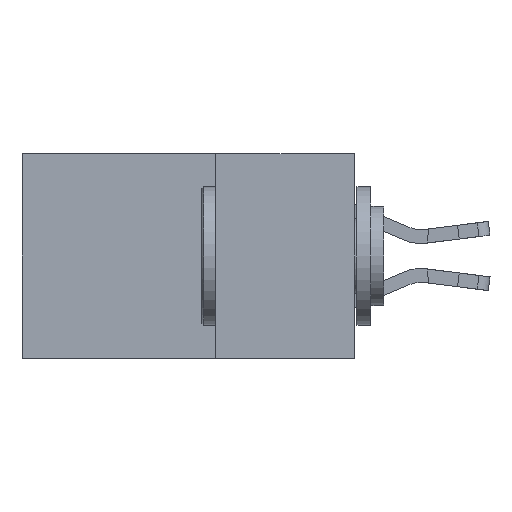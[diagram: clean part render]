
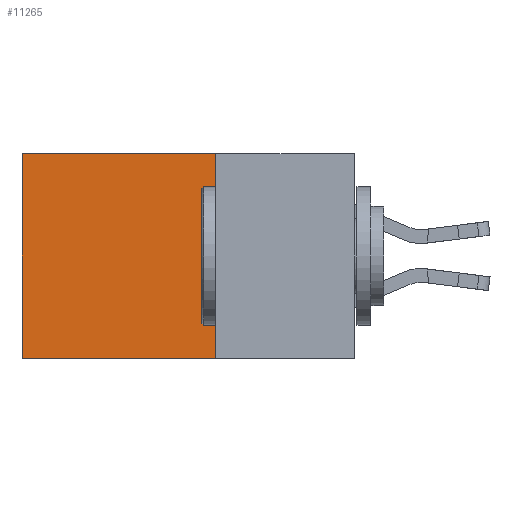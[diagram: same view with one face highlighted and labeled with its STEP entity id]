
A CAD part, left-side view. The second image highlights one B-rep face of the part: STEP entity #11265.
In plain terms, the highlighted planar face has unit normal (-1, 0, 0).
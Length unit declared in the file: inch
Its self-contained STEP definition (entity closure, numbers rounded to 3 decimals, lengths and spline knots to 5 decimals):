
#595 = VERTEX_POINT ( 'NONE', #12958 ) ;
#766 = AXIS2_PLACEMENT_3D ( 'NONE', #7417, #2821, #1043 ) ;
#771 = ORIENTED_EDGE ( 'NONE', *, *, #3186, .F. ) ;
#1043 = DIRECTION ( 'NONE',  ( 0., 0., -1. ) ) ;
#1897 = CARTESIAN_POINT ( 'NONE',  ( 0.298, 0.6, -0.37 ) ) ;
#2123 = EDGE_LOOP ( 'NONE', ( #4157, #17910, #771, #24128 ) ) ;
#2305 = CARTESIAN_POINT ( 'NONE',  ( 0.298, 0.25, 0. ) ) ;
#2821 = DIRECTION ( 'NONE',  ( 1., 0., 0. ) ) ;
#3186 = EDGE_CURVE ( 'NONE', #19483, #3662, #12262, .T. ) ;
#3662 = VERTEX_POINT ( 'NONE', #22411 ) ;
#3732 = EDGE_CURVE ( 'NONE', #595, #9090, #9239, .T. ) ;
#3915 = PLANE ( 'NONE',  #766 ) ;
#4157 = ORIENTED_EDGE ( 'NONE', *, *, #3732, .T. ) ;
#4269 = LINE ( 'NONE', #19987, #10978 ) ;
#4420 = CARTESIAN_POINT ( 'NONE',  ( 0.298, 0.6, 0. ) ) ;
#5191 = VECTOR ( 'NONE', #14835, 39.37008 ) ;
#6912 = VECTOR ( 'NONE', #19428, 39.37008 ) ;
#7417 = CARTESIAN_POINT ( 'NONE',  ( 0.298, 0.25, 0. ) ) ;
#9090 = VERTEX_POINT ( 'NONE', #1897 ) ;
#9239 = LINE ( 'NONE', #4420, #6912 ) ;
#9675 = EDGE_CURVE ( 'NONE', #19483, #595, #22666, .T. ) ;
#10978 = VECTOR ( 'NONE', #26471, 39.37008 ) ;
#11265 = ADVANCED_FACE ( 'NONE', ( #11778 ), #3915, .F. ) ;
#11778 = FACE_OUTER_BOUND ( 'NONE', #2123, .T. ) ;
#12262 = LINE ( 'NONE', #2305, #24087 ) ;
#12958 = CARTESIAN_POINT ( 'NONE',  ( 0.298, 0.6, 0. ) ) ;
#14835 = DIRECTION ( 'NONE',  ( 0., 1., 0. ) ) ;
#17910 = ORIENTED_EDGE ( 'NONE', *, *, #23928, .F. ) ;
#19428 = DIRECTION ( 'NONE',  ( 0., 0., -1. ) ) ;
#19483 = VERTEX_POINT ( 'NONE', #22305 ) ;
#19987 = CARTESIAN_POINT ( 'NONE',  ( 0.298, 0.25, -0.37 ) ) ;
#21726 = DIRECTION ( 'NONE',  ( 0., 0., -1. ) ) ;
#22305 = CARTESIAN_POINT ( 'NONE',  ( 0.298, 0.25, 0. ) ) ;
#22411 = CARTESIAN_POINT ( 'NONE',  ( 0.298, 0.25, -0.37 ) ) ;
#22666 = LINE ( 'NONE', #25615, #5191 ) ;
#23928 = EDGE_CURVE ( 'NONE', #3662, #9090, #4269, .T. ) ;
#24087 = VECTOR ( 'NONE', #21726, 39.37008 ) ;
#24128 = ORIENTED_EDGE ( 'NONE', *, *, #9675, .T. ) ;
#25615 = CARTESIAN_POINT ( 'NONE',  ( 0.298, 0.25, 0. ) ) ;
#26471 = DIRECTION ( 'NONE',  ( 0., 1., 0. ) ) ;
